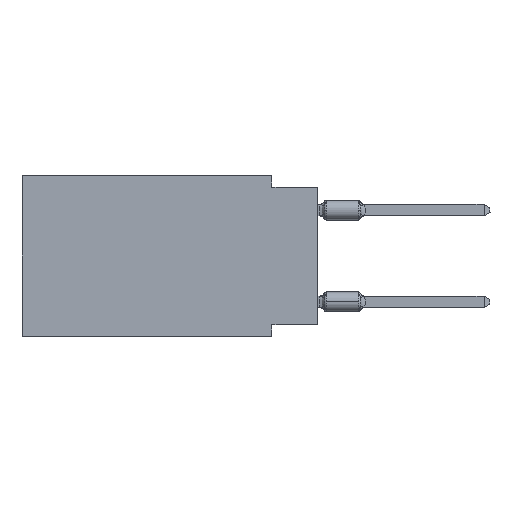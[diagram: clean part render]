
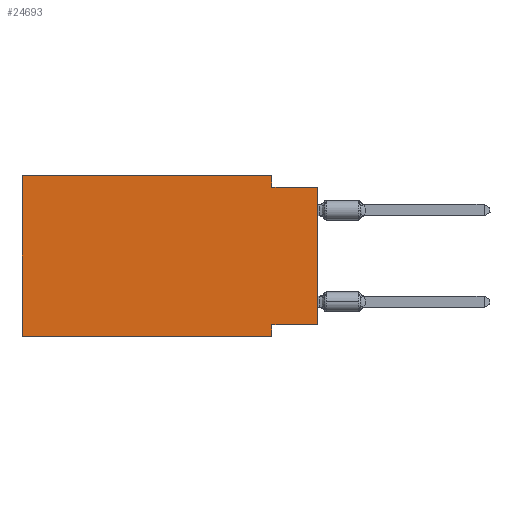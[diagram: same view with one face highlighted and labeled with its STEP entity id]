
A CAD part, left-side view. The second image highlights one B-rep face of the part: STEP entity #24693.
In plain terms, the highlighted planar face has unit normal (-1, 0, 0).
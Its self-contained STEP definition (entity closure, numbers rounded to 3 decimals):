
#391 = CARTESIAN_POINT ( 'NONE',  ( 0., 0., -8.255 ) ) ;
#1095 = VERTEX_POINT ( 'NONE', #2605 ) ;
#2605 = CARTESIAN_POINT ( 'NONE',  ( 0., 16.383, -8.89 ) ) ;
#3041 = VERTEX_POINT ( 'NONE', #41186 ) ;
#3445 = LINE ( 'NONE', #33333, #25051 ) ;
#3583 = VECTOR ( 'NONE', #43382, 1000. ) ;
#4628 = CARTESIAN_POINT ( 'NONE',  ( 0., 2.54, 0. ) ) ;
#6222 = ORIENTED_EDGE ( 'NONE', *, *, #15674, .F. ) ;
#7659 = LINE ( 'NONE', #32804, #37763 ) ;
#7716 = FACE_OUTER_BOUND ( 'NONE', #16449, .T. ) ;
#8000 = PLANE ( 'NONE',  #45674 ) ;
#8353 = EDGE_CURVE ( 'NONE', #30820, #29811, #51511, .T. ) ;
#9111 = LINE ( 'NONE', #47664, #32344 ) ;
#10259 = DIRECTION ( 'NONE',  ( 0., -1., 0. ) ) ;
#11265 = VERTEX_POINT ( 'NONE', #19398 ) ;
#11958 = ORIENTED_EDGE ( 'NONE', *, *, #42280, .F. ) ;
#12773 = EDGE_CURVE ( 'NONE', #29811, #26234, #23261, .T. ) ;
#15674 = EDGE_CURVE ( 'NONE', #22266, #11265, #9111, .T. ) ;
#16093 = DIRECTION ( 'NONE',  ( 0., 0., -1. ) ) ;
#16119 = DIRECTION ( 'NONE',  ( 1., 0., 0. ) ) ;
#16426 = VECTOR ( 'NONE', #54441, 1000. ) ;
#16449 = EDGE_LOOP ( 'NONE', ( #46885, #20246, #11958, #6222, #21452, #42721, #34490, #54218 ) ) ;
#16886 = VECTOR ( 'NONE', #19869, 1000. ) ;
#17000 = CARTESIAN_POINT ( 'NONE',  ( 0., 0., -0.635 ) ) ;
#17352 = EDGE_CURVE ( 'NONE', #22630, #3041, #33194, .T. ) ;
#17768 = DIRECTION ( 'NONE',  ( 0., -1., 0. ) ) ;
#19398 = CARTESIAN_POINT ( 'NONE',  ( 0., 2.54, 0. ) ) ;
#19869 = DIRECTION ( 'NONE',  ( 0., 0., 1. ) ) ;
#20200 = CARTESIAN_POINT ( 'NONE',  ( 0., 16.383, 0. ) ) ;
#20246 = ORIENTED_EDGE ( 'NONE', *, *, #17352, .F. ) ;
#20964 = CARTESIAN_POINT ( 'NONE',  ( 0., 2.54, -0.635 ) ) ;
#21452 = ORIENTED_EDGE ( 'NONE', *, *, #50138, .F. ) ;
#22266 = VERTEX_POINT ( 'NONE', #20200 ) ;
#22429 = VECTOR ( 'NONE', #35282, 1000. ) ;
#22630 = VERTEX_POINT ( 'NONE', #20964 ) ;
#23261 = LINE ( 'NONE', #36105, #22429 ) ;
#23504 = CARTESIAN_POINT ( 'NONE',  ( 0., 0., 0. ) ) ;
#24226 = CARTESIAN_POINT ( 'NONE',  ( 0., 16.383, 0. ) ) ;
#24693 = ADVANCED_FACE ( 'NONE', ( #7716 ), #8000, .F. ) ;
#25051 = VECTOR ( 'NONE', #10259, 1000. ) ;
#26234 = VERTEX_POINT ( 'NONE', #42372 ) ;
#28930 = LINE ( 'NONE', #4628, #47114 ) ;
#29811 = VERTEX_POINT ( 'NONE', #49267 ) ;
#30820 = VERTEX_POINT ( 'NONE', #47414 ) ;
#32344 = VECTOR ( 'NONE', #17768, 1000. ) ;
#32804 = CARTESIAN_POINT ( 'NONE',  ( 0., 16.383, 0. ) ) ;
#33194 = LINE ( 'NONE', #17000, #16426 ) ;
#33333 = CARTESIAN_POINT ( 'NONE',  ( 0., 16.383, -8.89 ) ) ;
#34490 = ORIENTED_EDGE ( 'NONE', *, *, #12773, .F. ) ;
#35282 = DIRECTION ( 'NONE',  ( 0., 0., -1. ) ) ;
#36048 = EDGE_CURVE ( 'NONE', #30820, #3041, #53402, .T. ) ;
#36105 = CARTESIAN_POINT ( 'NONE',  ( 0., 2.54, -8.89 ) ) ;
#36748 = DIRECTION ( 'NONE',  ( 0., 0., 1. ) ) ;
#37763 = VECTOR ( 'NONE', #36748, 1000. ) ;
#41186 = CARTESIAN_POINT ( 'NONE',  ( 0., 0., -0.635 ) ) ;
#42280 = EDGE_CURVE ( 'NONE', #11265, #22630, #28930, .T. ) ;
#42372 = CARTESIAN_POINT ( 'NONE',  ( 0., 2.54, -8.89 ) ) ;
#42721 = ORIENTED_EDGE ( 'NONE', *, *, #47473, .T. ) ;
#43382 = DIRECTION ( 'NONE',  ( 0., 1., 0. ) ) ;
#45674 = AXIS2_PLACEMENT_3D ( 'NONE', #24226, #16119, #54395 ) ;
#46885 = ORIENTED_EDGE ( 'NONE', *, *, #36048, .T. ) ;
#47114 = VECTOR ( 'NONE', #16093, 1000. ) ;
#47414 = CARTESIAN_POINT ( 'NONE',  ( 0., 0., -8.255 ) ) ;
#47473 = EDGE_CURVE ( 'NONE', #1095, #26234, #3445, .T. ) ;
#47664 = CARTESIAN_POINT ( 'NONE',  ( 0., 16.383, 0. ) ) ;
#49267 = CARTESIAN_POINT ( 'NONE',  ( 0., 2.54, -8.255 ) ) ;
#50138 = EDGE_CURVE ( 'NONE', #1095, #22266, #7659, .T. ) ;
#51511 = LINE ( 'NONE', #391, #3583 ) ;
#53402 = LINE ( 'NONE', #23504, #16886 ) ;
#54218 = ORIENTED_EDGE ( 'NONE', *, *, #8353, .F. ) ;
#54395 = DIRECTION ( 'NONE',  ( 0., 0., -1. ) ) ;
#54441 = DIRECTION ( 'NONE',  ( 0., -1., 0. ) ) ;
